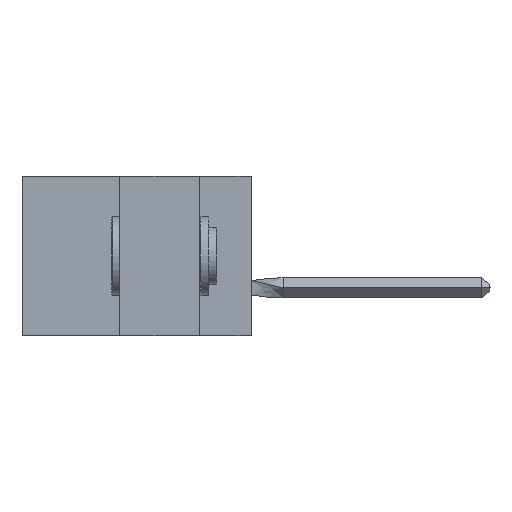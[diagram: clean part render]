
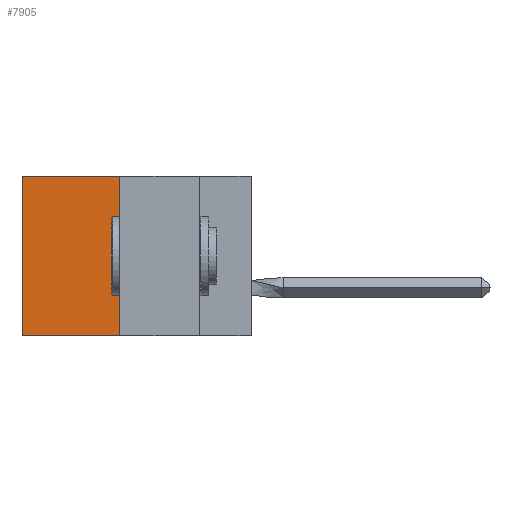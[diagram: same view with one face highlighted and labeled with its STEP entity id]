
A CAD part, left-side view. The second image highlights one B-rep face of the part: STEP entity #7905.
In plain terms, the highlighted planar face has unit normal (-1, 0, 0).
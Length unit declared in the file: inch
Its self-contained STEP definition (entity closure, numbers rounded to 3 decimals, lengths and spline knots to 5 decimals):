
#164 = CARTESIAN_POINT ( 'NONE',  ( 0.305, 0.413, -0.5 ) ) ;
#2337 = ORIENTED_EDGE ( 'NONE', *, *, #2812, .T. ) ;
#2812 = EDGE_CURVE ( 'NONE', #12255, #31826, #34134, .T. ) ;
#3742 = CARTESIAN_POINT ( 'NONE',  ( 0.305, 0.413, -0.5 ) ) ;
#4181 = EDGE_CURVE ( 'NONE', #35733, #12255, #8784, .T. ) ;
#4308 = VERTEX_POINT ( 'NONE', #164 ) ;
#5198 = VECTOR ( 'NONE', #18896, 39.37008 ) ;
#5704 = CARTESIAN_POINT ( 'NONE',  ( 0.305, 0.72, -0.5 ) ) ;
#6536 = DIRECTION ( 'NONE',  ( 0., 0., -1. ) ) ;
#7764 = ORIENTED_EDGE ( 'NONE', *, *, #10760, .F. ) ;
#7905 = ADVANCED_FACE ( 'NONE', ( #33730 ), #12149, .F. ) ;
#8628 = CARTESIAN_POINT ( 'NONE',  ( 0.305, 0.413, 0. ) ) ;
#8784 = LINE ( 'NONE', #27669, #31407 ) ;
#9775 = ORIENTED_EDGE ( 'NONE', *, *, #18905, .F. ) ;
#10487 = AXIS2_PLACEMENT_3D ( 'NONE', #3742, #23191, #6536 ) ;
#10760 = EDGE_CURVE ( 'NONE', #4308, #31826, #12616, .T. ) ;
#12149 = PLANE ( 'NONE',  #10487 ) ;
#12255 = VERTEX_POINT ( 'NONE', #32389 ) ;
#12616 = LINE ( 'NONE', #24569, #5198 ) ;
#16766 = VECTOR ( 'NONE', #30468, 39.37008 ) ;
#17692 = VECTOR ( 'NONE', #35960, 39.37008 ) ;
#18896 = DIRECTION ( 'NONE',  ( 0., 1., 0. ) ) ;
#18905 = EDGE_CURVE ( 'NONE', #35733, #4308, #33287, .T. ) ;
#23191 = DIRECTION ( 'NONE',  ( 1., 0., 0. ) ) ;
#24569 = CARTESIAN_POINT ( 'NONE',  ( 0.305, 0.413, -0.5 ) ) ;
#24656 = CARTESIAN_POINT ( 'NONE',  ( 0.305, 0.72, -0.5 ) ) ;
#25833 = EDGE_LOOP ( 'NONE', ( #2337, #7764, #9775, #35889 ) ) ;
#27669 = CARTESIAN_POINT ( 'NONE',  ( 0.305, 0.413, 0. ) ) ;
#30468 = DIRECTION ( 'NONE',  ( 0., 0., -1. ) ) ;
#31407 = VECTOR ( 'NONE', #33275, 39.37008 ) ;
#31826 = VERTEX_POINT ( 'NONE', #5704 ) ;
#32389 = CARTESIAN_POINT ( 'NONE',  ( 0.305, 0.72, 0. ) ) ;
#33275 = DIRECTION ( 'NONE',  ( 0., 1., 0. ) ) ;
#33287 = LINE ( 'NONE', #35458, #17692 ) ;
#33730 = FACE_OUTER_BOUND ( 'NONE', #25833, .T. ) ;
#34134 = LINE ( 'NONE', #24656, #16766 ) ;
#35458 = CARTESIAN_POINT ( 'NONE',  ( 0.305, 0.413, -0.5 ) ) ;
#35733 = VERTEX_POINT ( 'NONE', #8628 ) ;
#35889 = ORIENTED_EDGE ( 'NONE', *, *, #4181, .T. ) ;
#35960 = DIRECTION ( 'NONE',  ( 0., 0., -1. ) ) ;
